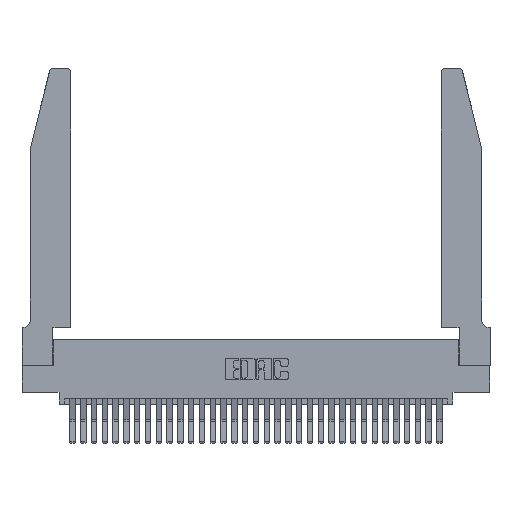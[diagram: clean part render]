
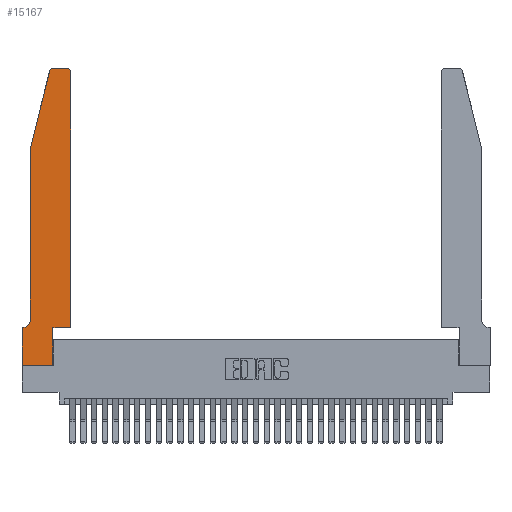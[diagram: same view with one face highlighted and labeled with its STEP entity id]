
A CAD part, top view. The second image highlights one B-rep face of the part: STEP entity #15167.
In plain terms, the highlighted planar face has unit normal (0, 0, 1).
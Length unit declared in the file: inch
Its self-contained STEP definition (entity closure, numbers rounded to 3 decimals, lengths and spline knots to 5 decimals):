
#217 = EDGE_CURVE ( 'NONE', #27802, #5872, #14018, .T. ) ;
#410 = DIRECTION ( 'NONE',  ( 0., 1., 0. ) ) ;
#684 = LINE ( 'NONE', #18471, #20597 ) ;
#989 = VECTOR ( 'NONE', #21674, 39.37008 ) ;
#1182 = VECTOR ( 'NONE', #18670, 39.37008 ) ;
#1191 = DIRECTION ( 'NONE',  ( 0., -1., 0. ) ) ;
#1569 = LINE ( 'NONE', #15082, #7798 ) ;
#3264 = ORIENTED_EDGE ( 'NONE', *, *, #19651, .T. ) ;
#3278 = LINE ( 'NONE', #10931, #9470 ) ;
#3792 = VECTOR ( 'NONE', #8131, 39.37008 ) ;
#3964 = LINE ( 'NONE', #7459, #16935 ) ;
#3979 = VERTEX_POINT ( 'NONE', #25138 ) ;
#4365 = CARTESIAN_POINT ( 'NONE',  ( 0.25487, 2.72718, 0.37 ) ) ;
#4568 = ORIENTED_EDGE ( 'NONE', *, *, #17193, .T. ) ;
#4713 = EDGE_CURVE ( 'NONE', #27264, #32230, #1569, .T. ) ;
#4822 = EDGE_CURVE ( 'NONE', #27166, #27802, #18239, .T. ) ;
#5124 = EDGE_CURVE ( 'NONE', #32230, #28034, #23832, .T. ) ;
#5350 = DIRECTION ( 'NONE',  ( 1., 0., 0. ) ) ;
#5451 = ORIENTED_EDGE ( 'NONE', *, *, #4822, .T. ) ;
#5872 = VERTEX_POINT ( 'NONE', #28728 ) ;
#6432 = DIRECTION ( 'NONE',  ( 0., 0., -1. ) ) ;
#6940 = CARTESIAN_POINT ( 'NONE',  ( 0.4205, 2.75, 0.37 ) ) ;
#7459 = CARTESIAN_POINT ( 'NONE',  ( 0., 0., 0.37 ) ) ;
#7463 = AXIS2_PLACEMENT_3D ( 'NONE', #7916, #25874, #10523 ) ;
#7714 = ORIENTED_EDGE ( 'NONE', *, *, #4713, .T. ) ;
#7798 = VECTOR ( 'NONE', #22866, 39.37008 ) ;
#7916 = CARTESIAN_POINT ( 'NONE',  ( 0.284, 2.72, 0.37 ) ) ;
#8107 = ORIENTED_EDGE ( 'NONE', *, *, #9373, .T. ) ;
#8131 = DIRECTION ( 'NONE',  ( 1., 0., 0. ) ) ;
#8358 = CARTESIAN_POINT ( 'NONE',  ( 0.0755, 0.42, 0.37 ) ) ;
#8405 = CARTESIAN_POINT ( 'NONE',  ( 0.4505, 0.35, 0.37 ) ) ;
#9373 = EDGE_CURVE ( 'NONE', #29918, #27944, #16750, .T. ) ;
#9466 = ORIENTED_EDGE ( 'NONE', *, *, #23615, .T. ) ;
#9470 = VECTOR ( 'NONE', #28820, 39.37008 ) ;
#9968 = ORIENTED_EDGE ( 'NONE', *, *, #14278, .T. ) ;
#10523 = DIRECTION ( 'NONE',  ( 1., 0., 0. ) ) ;
#10542 = EDGE_CURVE ( 'NONE', #5872, #25536, #3278, .T. ) ;
#10931 = CARTESIAN_POINT ( 'NONE',  ( 0.0755, 2., 0.37 ) ) ;
#11103 = DIRECTION ( 'NONE',  ( 0., 1., 0. ) ) ;
#11616 = CARTESIAN_POINT ( 'NONE',  ( 0., 0., 0.37 ) ) ;
#12716 = CARTESIAN_POINT ( 'NONE',  ( 0.0055, 0.35, 0.37 ) ) ;
#13219 = CIRCLE ( 'NONE', #30372, 0.07 ) ;
#13378 = CARTESIAN_POINT ( 'NONE',  ( 0., 0.35, 0.37 ) ) ;
#13664 = DIRECTION ( 'NONE',  ( 0., 0., 1. ) ) ;
#14018 = LINE ( 'NONE', #29236, #989 ) ;
#14278 = EDGE_CURVE ( 'NONE', #25536, #27264, #13219, .T. ) ;
#15076 = ORIENTED_EDGE ( 'NONE', *, *, #5124, .T. ) ;
#15082 = CARTESIAN_POINT ( 'NONE',  ( 0.0755, 0.35, 0.37 ) ) ;
#15167 = ADVANCED_FACE ( 'NONE', ( #18385 ), #15636, .T. ) ;
#15636 = PLANE ( 'NONE',  #21640 ) ;
#15860 = CARTESIAN_POINT ( 'NONE',  ( 0.4505, 0.35, 0.37 ) ) ;
#15934 = CARTESIAN_POINT ( 'NONE',  ( 0.2865, 0.35, 0.37 ) ) ;
#16682 = ORIENTED_EDGE ( 'NONE', *, *, #10542, .T. ) ;
#16750 = LINE ( 'NONE', #8405, #30358 ) ;
#16935 = VECTOR ( 'NONE', #25439, 39.37008 ) ;
#17193 = EDGE_CURVE ( 'NONE', #31219, #27166, #28629, .T. ) ;
#18233 = CARTESIAN_POINT ( 'NONE',  ( 0., 0.35, 0.37 ) ) ;
#18239 = CIRCLE ( 'NONE', #7463, 0.03 ) ;
#18385 = FACE_OUTER_BOUND ( 'NONE', #29399, .T. ) ;
#18471 = CARTESIAN_POINT ( 'NONE',  ( 0.2865, 0.35, 0.37 ) ) ;
#18670 = DIRECTION ( 'NONE',  ( -1., 0., 0. ) ) ;
#19217 = LINE ( 'NONE', #15860, #3792 ) ;
#19651 = EDGE_CURVE ( 'NONE', #27944, #31219, #32998, .T. ) ;
#19652 = CARTESIAN_POINT ( 'NONE',  ( 0.4505, 0.35, 0.37 ) ) ;
#20277 = EDGE_CURVE ( 'NONE', #3979, #26037, #684, .T. ) ;
#20597 = VECTOR ( 'NONE', #410, 39.37008 ) ;
#20817 = DIRECTION ( 'NONE',  ( 0., 0., 1. ) ) ;
#20881 = ORIENTED_EDGE ( 'NONE', *, *, #25322, .T. ) ;
#21111 = CARTESIAN_POINT ( 'NONE',  ( 0.4505, 2.72, 0.37 ) ) ;
#21640 = AXIS2_PLACEMENT_3D ( 'NONE', #18233, #20817, #5350 ) ;
#21674 = DIRECTION ( 'NONE',  ( -0.239, -0.971, 0. ) ) ;
#21869 = CARTESIAN_POINT ( 'NONE',  ( 0.0055, 0.42, 0.37 ) ) ;
#22866 = DIRECTION ( 'NONE',  ( -1., 0., 0. ) ) ;
#23615 = EDGE_CURVE ( 'NONE', #26037, #29918, #19217, .T. ) ;
#23832 = LINE ( 'NONE', #11616, #24636 ) ;
#24004 = CARTESIAN_POINT ( 'NONE',  ( 0., 0., 0.37 ) ) ;
#24425 = DIRECTION ( 'NONE',  ( -1., 0., 0. ) ) ;
#24636 = VECTOR ( 'NONE', #1191, 39.37008 ) ;
#25138 = CARTESIAN_POINT ( 'NONE',  ( 0.2865, 0., 0.37 ) ) ;
#25322 = EDGE_CURVE ( 'NONE', #28034, #3979, #3964, .T. ) ;
#25439 = DIRECTION ( 'NONE',  ( 1., 0., 0. ) ) ;
#25536 = VERTEX_POINT ( 'NONE', #8358 ) ;
#25874 = DIRECTION ( 'NONE',  ( 0., 0., 1. ) ) ;
#26037 = VERTEX_POINT ( 'NONE', #15934 ) ;
#27166 = VERTEX_POINT ( 'NONE', #29952 ) ;
#27264 = VERTEX_POINT ( 'NONE', #12716 ) ;
#27490 = AXIS2_PLACEMENT_3D ( 'NONE', #29006, #13664, #31567 ) ;
#27802 = VERTEX_POINT ( 'NONE', #4365 ) ;
#27944 = VERTEX_POINT ( 'NONE', #21111 ) ;
#28034 = VERTEX_POINT ( 'NONE', #24004 ) ;
#28629 = LINE ( 'NONE', #31400, #1182 ) ;
#28728 = CARTESIAN_POINT ( 'NONE',  ( 0.0755, 2., 0.37 ) ) ;
#28820 = DIRECTION ( 'NONE',  ( 0., -1., 0. ) ) ;
#29006 = CARTESIAN_POINT ( 'NONE',  ( 0.4205, 2.72, 0.37 ) ) ;
#29065 = ORIENTED_EDGE ( 'NONE', *, *, #20277, .T. ) ;
#29236 = CARTESIAN_POINT ( 'NONE',  ( 0.0755, 2., 0.37 ) ) ;
#29399 = EDGE_LOOP ( 'NONE', ( #4568, #5451, #30932, #16682, #9968, #7714, #15076, #20881, #29065, #9466, #8107, #3264 ) ) ;
#29918 = VERTEX_POINT ( 'NONE', #19652 ) ;
#29952 = CARTESIAN_POINT ( 'NONE',  ( 0.284, 2.75, 0.37 ) ) ;
#30358 = VECTOR ( 'NONE', #11103, 39.37008 ) ;
#30372 = AXIS2_PLACEMENT_3D ( 'NONE', #21869, #6432, #24425 ) ;
#30932 = ORIENTED_EDGE ( 'NONE', *, *, #217, .T. ) ;
#31219 = VERTEX_POINT ( 'NONE', #6940 ) ;
#31400 = CARTESIAN_POINT ( 'NONE',  ( 0.2605, 2.75, 0.37 ) ) ;
#31567 = DIRECTION ( 'NONE',  ( 1., 0., 0. ) ) ;
#32230 = VERTEX_POINT ( 'NONE', #13378 ) ;
#32998 = CIRCLE ( 'NONE', #27490, 0.03 ) ;
